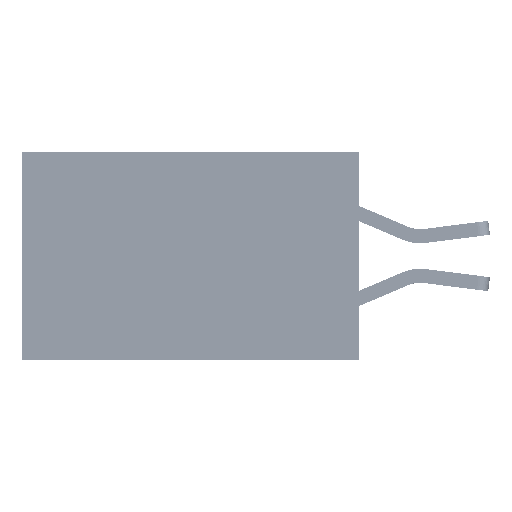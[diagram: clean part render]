
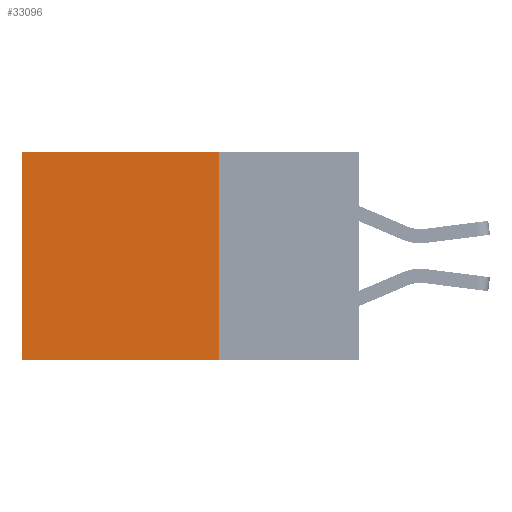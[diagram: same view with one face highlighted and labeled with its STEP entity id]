
A CAD part, left-side view. The second image highlights one B-rep face of the part: STEP entity #33096.
In plain terms, the highlighted planar face has unit normal (-1, 0, 0).
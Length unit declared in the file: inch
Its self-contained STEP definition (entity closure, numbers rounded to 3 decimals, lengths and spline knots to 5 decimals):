
#4342 = EDGE_CURVE ( 'NONE', #34324, #16642, #36761, .T. ) ;
#4785 = FACE_OUTER_BOUND ( 'NONE', #31356, .T. ) ;
#5218 = EDGE_CURVE ( 'NONE', #16642, #22893, #42387, .T. ) ;
#5848 = CARTESIAN_POINT ( 'NONE',  ( 0.2875, 0.25, 0. ) ) ;
#8728 = CARTESIAN_POINT ( 'NONE',  ( 0.2875, 0.25, 0. ) ) ;
#13315 = DIRECTION ( 'NONE',  ( 0., 0., -1. ) ) ;
#14735 = DIRECTION ( 'NONE',  ( 1., 0., 0. ) ) ;
#14945 = EDGE_CURVE ( 'NONE', #34324, #22630, #26918, .T. ) ;
#16642 = VERTEX_POINT ( 'NONE', #36968 ) ;
#16780 = VECTOR ( 'NONE', #13315, 39.37008 ) ;
#17425 = ORIENTED_EDGE ( 'NONE', *, *, #5218, .F. ) ;
#18220 = VECTOR ( 'NONE', #40875, 39.37008 ) ;
#19096 = AXIS2_PLACEMENT_3D ( 'NONE', #8728, #14735, #31189 ) ;
#21449 = CARTESIAN_POINT ( 'NONE',  ( 0.2875, 0.6, 0. ) ) ;
#22630 = VERTEX_POINT ( 'NONE', #21449 ) ;
#22893 = VERTEX_POINT ( 'NONE', #37426 ) ;
#25599 = DIRECTION ( 'NONE',  ( 0., 0., -1. ) ) ;
#26918 = LINE ( 'NONE', #30967, #18220 ) ;
#27244 = CARTESIAN_POINT ( 'NONE',  ( 0.2875, 0.25, 0. ) ) ;
#27527 = VECTOR ( 'NONE', #36380, 39.37008 ) ;
#28352 = PLANE ( 'NONE',  #19096 ) ;
#29812 = CARTESIAN_POINT ( 'NONE',  ( 0.2875, 0.25, -0.37 ) ) ;
#30320 = VECTOR ( 'NONE', #25599, 39.37008 ) ;
#30568 = ORIENTED_EDGE ( 'NONE', *, *, #14945, .T. ) ;
#30967 = CARTESIAN_POINT ( 'NONE',  ( 0.2875, 0.25, 0. ) ) ;
#31189 = DIRECTION ( 'NONE',  ( 0., 0., -1. ) ) ;
#31356 = EDGE_LOOP ( 'NONE', ( #33133, #17425, #40105, #30568 ) ) ;
#33096 = ADVANCED_FACE ( 'NONE', ( #4785 ), #28352, .F. ) ;
#33133 = ORIENTED_EDGE ( 'NONE', *, *, #41899, .T. ) ;
#34324 = VERTEX_POINT ( 'NONE', #5848 ) ;
#35462 = LINE ( 'NONE', #38897, #30320 ) ;
#36380 = DIRECTION ( 'NONE',  ( 0., 1., 0. ) ) ;
#36761 = LINE ( 'NONE', #27244, #16780 ) ;
#36968 = CARTESIAN_POINT ( 'NONE',  ( 0.2875, 0.25, -0.37 ) ) ;
#37426 = CARTESIAN_POINT ( 'NONE',  ( 0.2875, 0.6, -0.37 ) ) ;
#38897 = CARTESIAN_POINT ( 'NONE',  ( 0.2875, 0.6, 0. ) ) ;
#40105 = ORIENTED_EDGE ( 'NONE', *, *, #4342, .F. ) ;
#40875 = DIRECTION ( 'NONE',  ( 0., 1., 0. ) ) ;
#41899 = EDGE_CURVE ( 'NONE', #22630, #22893, #35462, .T. ) ;
#42387 = LINE ( 'NONE', #29812, #27527 ) ;
